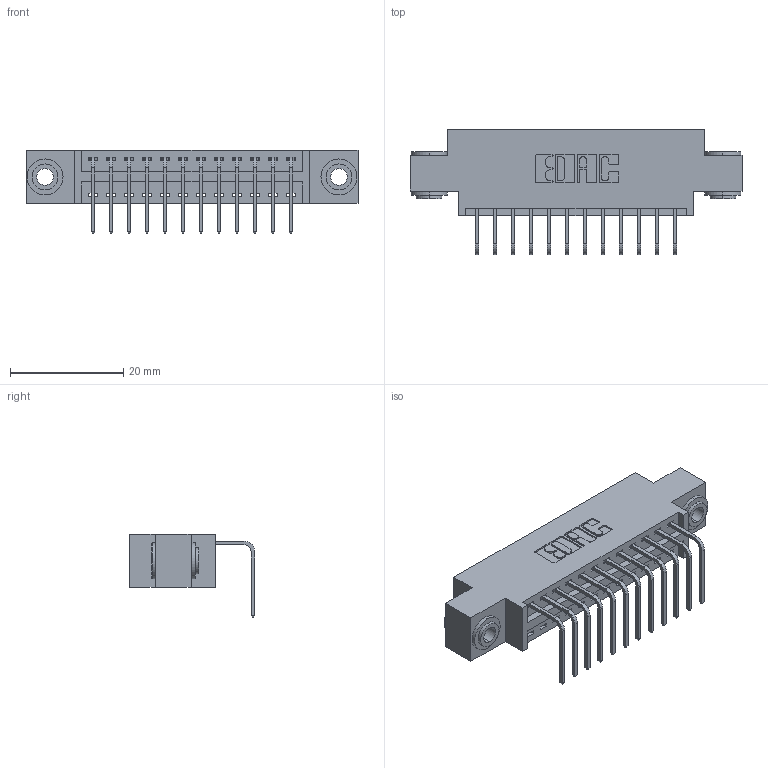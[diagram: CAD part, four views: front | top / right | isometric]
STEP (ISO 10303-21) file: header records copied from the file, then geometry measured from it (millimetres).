
FILE_DESCRIPTION (( 'STEP AP203' ), '1' );
FILE_NAME ('346-012-558-603.STEP', '2022-05-05T03:26:27', ( '' ), ( '' ), 'SwSTEP 2.0', 'SolidWorks 2020', '' );
FILE_SCHEMA (( 'CONFIG_CONTROL_DESIGN' ));
Length unit declared in the file: inch
Products named in the file (4): 346 Part_0.170 Offset - 0.156 Dia-TH; 345-292-001_558 Tail - 2; 346-012-558-603; 345-250-002_345-250-002-102
Assembly tree (15 placements, depth 2):
  346-012-558-603
    346 Part_0.170 Offset - 0.156 Dia-TH
    345-292-001_558 Tail - 2  x12
    345-250-002_345-250-002-102  x2
Bounding box: 58.67 x 22.16 x 14.73 mm (x, y, z)
Volume: 5296.4 mm3; surface area: 6946.4 mm2
Topology: 15 solids, 15 shells, 898 faces, 2637 edges, 1738 vertices
Faces by surface type: plane 608, cylinder 282, cone 8
Entity records: 12768 total; most frequent: CARTESIAN_POINT 2181, ORIENTED_EDGE 2118, DIRECTION 1989, EDGE_CURVE 1059, VECTOR 855, LINE 855, VERTEX_POINT 702, AXIS2_PLACEMENT_3D 567
